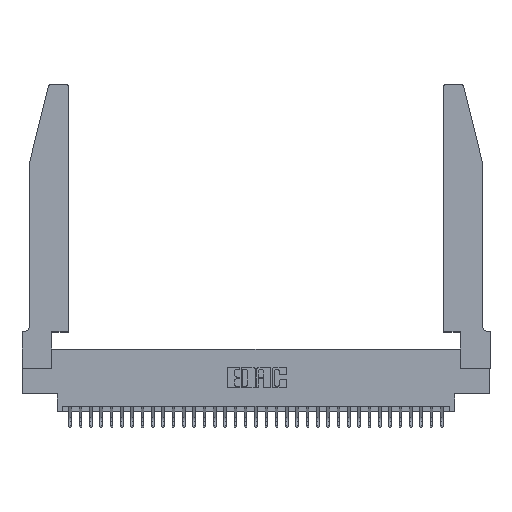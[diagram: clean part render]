
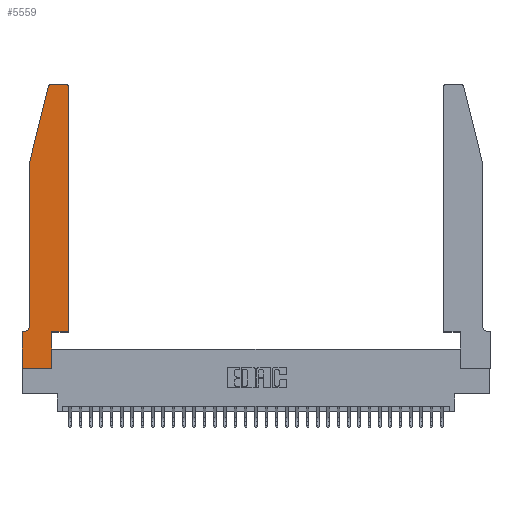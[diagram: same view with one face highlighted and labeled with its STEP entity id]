
A CAD part, top view. The second image highlights one B-rep face of the part: STEP entity #5559.
In plain terms, the highlighted planar face has unit normal (0, 0, 1).
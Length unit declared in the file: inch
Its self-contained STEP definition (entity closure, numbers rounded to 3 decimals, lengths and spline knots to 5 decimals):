
#511 = EDGE_CURVE ( 'NONE', #31018, #6737, #30341, .T. ) ;
#1307 = CARTESIAN_POINT ( 'NONE',  ( 0.4505, 0.35, 0.37 ) ) ;
#1935 = DIRECTION ( 'NONE',  ( 1., 0., 0. ) ) ;
#1972 = ORIENTED_EDGE ( 'NONE', *, *, #7586, .T. ) ;
#2112 = ORIENTED_EDGE ( 'NONE', *, *, #511, .T. ) ;
#2369 = DIRECTION ( 'NONE',  ( 0., -1., 0. ) ) ;
#2521 = LINE ( 'NONE', #26903, #10693 ) ;
#2681 = CARTESIAN_POINT ( 'NONE',  ( 0.2605, 2.75, 0.37 ) ) ;
#2857 = VECTOR ( 'NONE', #21117, 39.37008 ) ;
#2913 = DIRECTION ( 'NONE',  ( -1., 0., 0. ) ) ;
#2915 = VERTEX_POINT ( 'NONE', #29068 ) ;
#3383 = CARTESIAN_POINT ( 'NONE',  ( 0.284, 2.72, 0.37 ) ) ;
#3474 = CARTESIAN_POINT ( 'NONE',  ( 0.4205, 2.72, 0.37 ) ) ;
#3538 = ORIENTED_EDGE ( 'NONE', *, *, #24021, .T. ) ;
#3908 = CARTESIAN_POINT ( 'NONE',  ( 0., 0.35, 0.37 ) ) ;
#4087 = ORIENTED_EDGE ( 'NONE', *, *, #18319, .T. ) ;
#4108 = VECTOR ( 'NONE', #7982, 39.37008 ) ;
#4619 = AXIS2_PLACEMENT_3D ( 'NONE', #3474, #22318, #6263 ) ;
#5321 = DIRECTION ( 'NONE',  ( 1., 0., 0. ) ) ;
#5559 = ADVANCED_FACE ( 'NONE', ( #20070 ), #27125, .T. ) ;
#5700 = CARTESIAN_POINT ( 'NONE',  ( 0.0755, 0.35, 0.37 ) ) ;
#5784 = VERTEX_POINT ( 'NONE', #25490 ) ;
#5927 = ORIENTED_EDGE ( 'NONE', *, *, #27928, .T. ) ;
#6049 = LINE ( 'NONE', #22412, #26563 ) ;
#6113 = LINE ( 'NONE', #6178, #33671 ) ;
#6173 = DIRECTION ( 'NONE',  ( 1., 0., 0. ) ) ;
#6178 = CARTESIAN_POINT ( 'NONE',  ( 0.4505, 0.35, 0.37 ) ) ;
#6263 = DIRECTION ( 'NONE',  ( 1., 0., 0. ) ) ;
#6393 = AXIS2_PLACEMENT_3D ( 'NONE', #3383, #22231, #6173 ) ;
#6727 = VERTEX_POINT ( 'NONE', #14680 ) ;
#6737 = VERTEX_POINT ( 'NONE', #3908 ) ;
#7236 = EDGE_CURVE ( 'NONE', #31415, #28206, #6113, .T. ) ;
#7565 = DIRECTION ( 'NONE',  ( 0., 0., -1. ) ) ;
#7586 = EDGE_CURVE ( 'NONE', #5784, #31018, #9486, .T. ) ;
#7982 = DIRECTION ( 'NONE',  ( -1., 0., 0. ) ) ;
#8208 = DIRECTION ( 'NONE',  ( 0., 1., 0. ) ) ;
#8234 = ORIENTED_EDGE ( 'NONE', *, *, #31754, .T. ) ;
#8678 = AXIS2_PLACEMENT_3D ( 'NONE', #23574, #7565, #26286 ) ;
#9079 = VECTOR ( 'NONE', #2913, 39.37008 ) ;
#9486 = CIRCLE ( 'NONE', #8678, 0.07 ) ;
#9650 = ORIENTED_EDGE ( 'NONE', *, *, #17929, .T. ) ;
#10216 = VERTEX_POINT ( 'NONE', #16483 ) ;
#10693 = VECTOR ( 'NONE', #8208, 39.37008 ) ;
#10997 = LINE ( 'NONE', #23657, #2857 ) ;
#11204 = ORIENTED_EDGE ( 'NONE', *, *, #15718, .T. ) ;
#11635 = ORIENTED_EDGE ( 'NONE', *, *, #30640, .T. ) ;
#11641 = ORIENTED_EDGE ( 'NONE', *, *, #29122, .T. ) ;
#13816 = CARTESIAN_POINT ( 'NONE',  ( 0., 0.35, 0.37 ) ) ;
#14339 = CARTESIAN_POINT ( 'NONE',  ( 0.4505, 2.72, 0.37 ) ) ;
#14680 = CARTESIAN_POINT ( 'NONE',  ( 0.2865, 0., 0.37 ) ) ;
#15170 = CARTESIAN_POINT ( 'NONE',  ( 0.25487, 2.72718, 0.37 ) ) ;
#15437 = VECTOR ( 'NONE', #2369, 39.37008 ) ;
#15465 = LINE ( 'NONE', #29403, #27975 ) ;
#15718 = EDGE_CURVE ( 'NONE', #10216, #5784, #6049, .T. ) ;
#16483 = CARTESIAN_POINT ( 'NONE',  ( 0.0755, 2., 0.37 ) ) ;
#16520 = DIRECTION ( 'NONE',  ( 1., 0., 0. ) ) ;
#17524 = LINE ( 'NONE', #18194, #30822 ) ;
#17929 = EDGE_CURVE ( 'NONE', #22989, #22158, #32592, .T. ) ;
#18059 = AXIS2_PLACEMENT_3D ( 'NONE', #13816, #32439, #16520 ) ;
#18194 = CARTESIAN_POINT ( 'NONE',  ( 0.4505, 0.35, 0.37 ) ) ;
#18274 = CIRCLE ( 'NONE', #4619, 0.03 ) ;
#18319 = EDGE_CURVE ( 'NONE', #22158, #19216, #34215, .T. ) ;
#19216 = VERTEX_POINT ( 'NONE', #15170 ) ;
#19297 = EDGE_CURVE ( 'NONE', #30993, #31415, #17524, .T. ) ;
#19301 = ORIENTED_EDGE ( 'NONE', *, *, #19297, .T. ) ;
#19701 = ORIENTED_EDGE ( 'NONE', *, *, #7236, .T. ) ;
#20070 = FACE_OUTER_BOUND ( 'NONE', #20614, .T. ) ;
#20614 = EDGE_LOOP ( 'NONE', ( #9650, #4087, #5927, #11204, #1972, #2112, #3538, #11641, #8234, #19301, #19701, #11635 ) ) ;
#21117 = DIRECTION ( 'NONE',  ( -0.239, -0.971, 0. ) ) ;
#22158 = VERTEX_POINT ( 'NONE', #27371 ) ;
#22231 = DIRECTION ( 'NONE',  ( 0., 0., 1. ) ) ;
#22318 = DIRECTION ( 'NONE',  ( 0., 0., 1. ) ) ;
#22412 = CARTESIAN_POINT ( 'NONE',  ( 0.0755, 2., 0.37 ) ) ;
#22989 = VERTEX_POINT ( 'NONE', #25236 ) ;
#23574 = CARTESIAN_POINT ( 'NONE',  ( 0.0055, 0.42, 0.37 ) ) ;
#23657 = CARTESIAN_POINT ( 'NONE',  ( 0.0755, 2., 0.37 ) ) ;
#24021 = EDGE_CURVE ( 'NONE', #6737, #2915, #28778, .T. ) ;
#24907 = DIRECTION ( 'NONE',  ( 0., 1., 0. ) ) ;
#25086 = DIRECTION ( 'NONE',  ( 0., -1., 0. ) ) ;
#25236 = CARTESIAN_POINT ( 'NONE',  ( 0.4205, 2.75, 0.37 ) ) ;
#25490 = CARTESIAN_POINT ( 'NONE',  ( 0.0755, 0.42, 0.37 ) ) ;
#26286 = DIRECTION ( 'NONE',  ( -1., 0., 0. ) ) ;
#26374 = CARTESIAN_POINT ( 'NONE',  ( 0.0055, 0.35, 0.37 ) ) ;
#26563 = VECTOR ( 'NONE', #25086, 39.37008 ) ;
#26634 = CARTESIAN_POINT ( 'NONE',  ( 0., 0., 0.37 ) ) ;
#26903 = CARTESIAN_POINT ( 'NONE',  ( 0.2865, 0.35, 0.37 ) ) ;
#27125 = PLANE ( 'NONE',  #18059 ) ;
#27371 = CARTESIAN_POINT ( 'NONE',  ( 0.284, 2.75, 0.37 ) ) ;
#27928 = EDGE_CURVE ( 'NONE', #19216, #10216, #10997, .T. ) ;
#27975 = VECTOR ( 'NONE', #5321, 39.37008 ) ;
#28206 = VERTEX_POINT ( 'NONE', #14339 ) ;
#28778 = LINE ( 'NONE', #26634, #15437 ) ;
#28804 = CARTESIAN_POINT ( 'NONE',  ( 0.2865, 0.35, 0.37 ) ) ;
#29068 = CARTESIAN_POINT ( 'NONE',  ( 0., 0., 0.37 ) ) ;
#29122 = EDGE_CURVE ( 'NONE', #2915, #6727, #15465, .T. ) ;
#29403 = CARTESIAN_POINT ( 'NONE',  ( 0., 0., 0.37 ) ) ;
#30341 = LINE ( 'NONE', #5700, #9079 ) ;
#30640 = EDGE_CURVE ( 'NONE', #28206, #22989, #18274, .T. ) ;
#30822 = VECTOR ( 'NONE', #1935, 39.37008 ) ;
#30993 = VERTEX_POINT ( 'NONE', #28804 ) ;
#31018 = VERTEX_POINT ( 'NONE', #26374 ) ;
#31415 = VERTEX_POINT ( 'NONE', #1307 ) ;
#31754 = EDGE_CURVE ( 'NONE', #6727, #30993, #2521, .T. ) ;
#32439 = DIRECTION ( 'NONE',  ( 0., 0., 1. ) ) ;
#32592 = LINE ( 'NONE', #2681, #4108 ) ;
#33671 = VECTOR ( 'NONE', #24907, 39.37008 ) ;
#34215 = CIRCLE ( 'NONE', #6393, 0.03 ) ;
